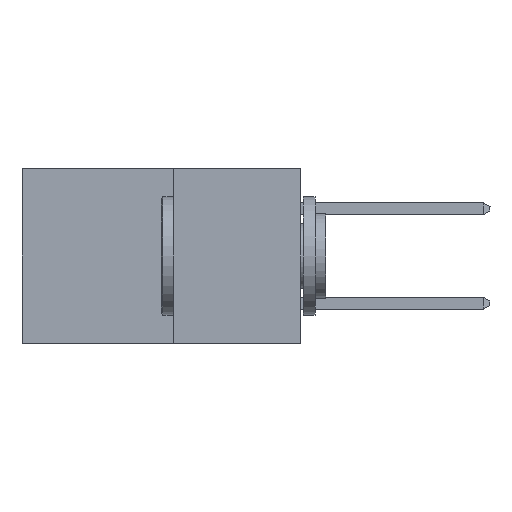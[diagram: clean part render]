
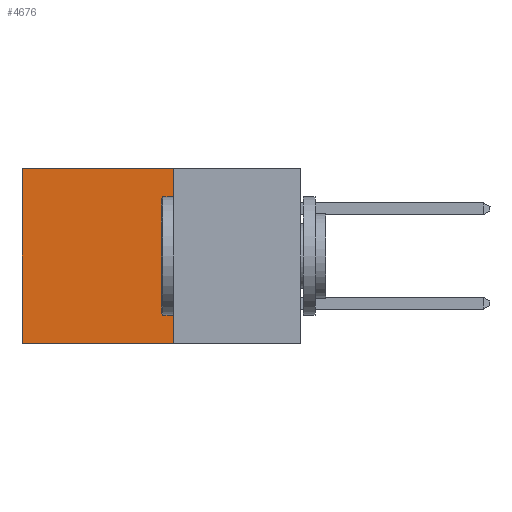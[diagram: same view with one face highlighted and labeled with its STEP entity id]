
A CAD part, left-side view. The second image highlights one B-rep face of the part: STEP entity #4676.
In plain terms, the highlighted planar face has unit normal (-1, 0, 0).
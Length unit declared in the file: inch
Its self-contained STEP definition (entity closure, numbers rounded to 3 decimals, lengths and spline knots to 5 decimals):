
#90 = CARTESIAN_POINT ( 'NONE',  ( 0.277, 0.59, 0. ) ) ;
#99 = CARTESIAN_POINT ( 'NONE',  ( 0.277, 0.27, -0.37 ) ) ;
#1137 = VECTOR ( 'NONE', #6658, 39.37008 ) ;
#1709 = CARTESIAN_POINT ( 'NONE',  ( 0.277, 0.27, 0. ) ) ;
#2310 = EDGE_CURVE ( 'NONE', #6993, #11887, #11158, .T. ) ;
#2356 = ORIENTED_EDGE ( 'NONE', *, *, #2310, .T. ) ;
#2737 = EDGE_LOOP ( 'NONE', ( #2356, #4302, #4345, #6238 ) ) ;
#3103 = CARTESIAN_POINT ( 'NONE',  ( 0.277, 0.59, -0.37 ) ) ;
#3174 = CARTESIAN_POINT ( 'NONE',  ( 0.277, 0.27, -0.37 ) ) ;
#3700 = FACE_OUTER_BOUND ( 'NONE', #2737, .T. ) ;
#4302 = ORIENTED_EDGE ( 'NONE', *, *, #12614, .F. ) ;
#4345 = ORIENTED_EDGE ( 'NONE', *, *, #6035, .F. ) ;
#4539 = DIRECTION ( 'NONE',  ( 0., 0., -1. ) ) ;
#4594 = DIRECTION ( 'NONE',  ( 1., 0., 0. ) ) ;
#4676 = ADVANCED_FACE ( 'NONE', ( #3700 ), #6366, .F. ) ;
#4849 = CARTESIAN_POINT ( 'NONE',  ( 0.277, 0.27, -0.37 ) ) ;
#5215 = VECTOR ( 'NONE', #6703, 39.37008 ) ;
#6035 = EDGE_CURVE ( 'NONE', #10386, #8067, #6762, .T. ) ;
#6238 = ORIENTED_EDGE ( 'NONE', *, *, #11766, .T. ) ;
#6366 = PLANE ( 'NONE',  #13465 ) ;
#6377 = CARTESIAN_POINT ( 'NONE',  ( 0.277, 0.59, -0.37 ) ) ;
#6606 = LINE ( 'NONE', #9211, #12234 ) ;
#6647 = CARTESIAN_POINT ( 'NONE',  ( 0.277, 0.27, -0.37 ) ) ;
#6658 = DIRECTION ( 'NONE',  ( 0., 0., -1. ) ) ;
#6703 = DIRECTION ( 'NONE',  ( 0., 0., -1. ) ) ;
#6762 = LINE ( 'NONE', #6647, #1137 ) ;
#6993 = VERTEX_POINT ( 'NONE', #90 ) ;
#8067 = VERTEX_POINT ( 'NONE', #99 ) ;
#9211 = CARTESIAN_POINT ( 'NONE',  ( 0.277, 0.27, 0. ) ) ;
#9469 = DIRECTION ( 'NONE',  ( 0., 1., 0. ) ) ;
#9691 = VECTOR ( 'NONE', #9469, 39.37008 ) ;
#10304 = DIRECTION ( 'NONE',  ( 0., 1., 0. ) ) ;
#10386 = VERTEX_POINT ( 'NONE', #1709 ) ;
#11158 = LINE ( 'NONE', #6377, #5215 ) ;
#11766 = EDGE_CURVE ( 'NONE', #10386, #6993, #6606, .T. ) ;
#11887 = VERTEX_POINT ( 'NONE', #3103 ) ;
#12234 = VECTOR ( 'NONE', #10304, 39.37008 ) ;
#12614 = EDGE_CURVE ( 'NONE', #8067, #11887, #13471, .T. ) ;
#13465 = AXIS2_PLACEMENT_3D ( 'NONE', #4849, #4594, #4539 ) ;
#13471 = LINE ( 'NONE', #3174, #9691 ) ;
